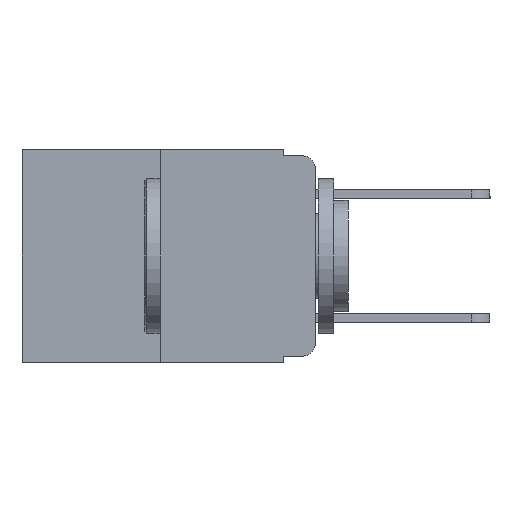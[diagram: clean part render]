
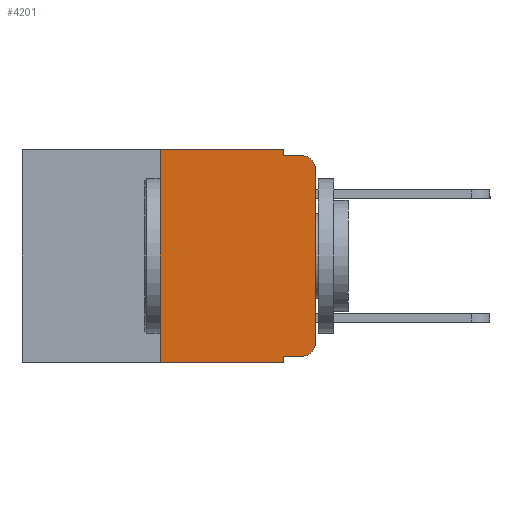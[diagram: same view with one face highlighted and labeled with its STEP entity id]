
A CAD part, left-side view. The second image highlights one B-rep face of the part: STEP entity #4201.
In plain terms, the highlighted planar face has unit normal (-1, 0, 0).
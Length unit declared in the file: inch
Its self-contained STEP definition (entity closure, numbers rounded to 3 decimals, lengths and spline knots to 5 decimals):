
#99 = DIRECTION ( 'NONE',  ( 0., -1., 0. ) ) ;
#253 = DIRECTION ( 'NONE',  ( -1., 0., 0. ) ) ;
#436 = CARTESIAN_POINT ( 'NONE',  ( 0., 0.02, -0.03 ) ) ;
#542 = ORIENTED_EDGE ( 'NONE', *, *, #10920, .F. ) ;
#738 = CARTESIAN_POINT ( 'NONE',  ( 0., 0.051, 0. ) ) ;
#1209 = CARTESIAN_POINT ( 'NONE',  ( 0., 0.473, -0.343 ) ) ;
#1216 = CARTESIAN_POINT ( 'NONE',  ( 0., 0.02, -0.01 ) ) ;
#1222 = DIRECTION ( 'NONE',  ( 0., 0., -1. ) ) ;
#1308 = ORIENTED_EDGE ( 'NONE', *, *, #7021, .T. ) ;
#1904 = LINE ( 'NONE', #7914, #5536 ) ;
#2369 = CARTESIAN_POINT ( 'NONE',  ( 0., 0.051, 0. ) ) ;
#2874 = CARTESIAN_POINT ( 'NONE',  ( 0., 0.02, -0.313 ) ) ;
#2912 = AXIS2_PLACEMENT_3D ( 'NONE', #436, #253, #1222 ) ;
#3147 = ORIENTED_EDGE ( 'NONE', *, *, #16423, .F. ) ;
#3203 = ORIENTED_EDGE ( 'NONE', *, *, #19308, .F. ) ;
#3329 = VECTOR ( 'NONE', #14555, 39.37008 ) ;
#3749 = EDGE_CURVE ( 'NONE', #11723, #16926, #11195, .T. ) ;
#3936 = DIRECTION ( 'NONE',  ( 0., -1., 0. ) ) ;
#4201 = ADVANCED_FACE ( 'NONE', ( #15948 ), #7211, .F. ) ;
#4256 = ORIENTED_EDGE ( 'NONE', *, *, #14523, .T. ) ;
#4447 = DIRECTION ( 'NONE',  ( 0., 0., -1. ) ) ;
#4767 = AXIS2_PLACEMENT_3D ( 'NONE', #2874, #13539, #4447 ) ;
#5006 = CIRCLE ( 'NONE', #2912, 0.02 ) ;
#5343 = ORIENTED_EDGE ( 'NONE', *, *, #10565, .F. ) ;
#5536 = VECTOR ( 'NONE', #99, 39.37008 ) ;
#5623 = ORIENTED_EDGE ( 'NONE', *, *, #9549, .T. ) ;
#5630 = ORIENTED_EDGE ( 'NONE', *, *, #7796, .T. ) ;
#5856 = VERTEX_POINT ( 'NONE', #1216 ) ;
#6713 = AXIS2_PLACEMENT_3D ( 'NONE', #8072, #7779, #13827 ) ;
#6740 = DIRECTION ( 'NONE',  ( 0., -1., 0. ) ) ;
#7021 = EDGE_CURVE ( 'NONE', #16243, #13256, #19217, .T. ) ;
#7211 = PLANE ( 'NONE',  #6713 ) ;
#7239 = VERTEX_POINT ( 'NONE', #8903 ) ;
#7547 = VERTEX_POINT ( 'NONE', #18936 ) ;
#7779 = DIRECTION ( 'NONE',  ( 1., 0., 0. ) ) ;
#7796 = EDGE_CURVE ( 'NONE', #13256, #5856, #5006, .T. ) ;
#7892 = VECTOR ( 'NONE', #10334, 39.37008 ) ;
#7914 = CARTESIAN_POINT ( 'NONE',  ( 0., 0.473, 0. ) ) ;
#8072 = CARTESIAN_POINT ( 'NONE',  ( 0., 0.473, 0. ) ) ;
#8608 = ORIENTED_EDGE ( 'NONE', *, *, #3749, .T. ) ;
#8821 = ORIENTED_EDGE ( 'NONE', *, *, #18351, .F. ) ;
#8903 = CARTESIAN_POINT ( 'NONE',  ( 0., 0.051, -0.01 ) ) ;
#9040 = VECTOR ( 'NONE', #12031, 39.37008 ) ;
#9549 = EDGE_CURVE ( 'NONE', #10768, #16243, #13540, .T. ) ;
#10184 = CARTESIAN_POINT ( 'NONE',  ( 0., 0., 0. ) ) ;
#10334 = DIRECTION ( 'NONE',  ( 0., 0., 1. ) ) ;
#10517 = CARTESIAN_POINT ( 'NONE',  ( 0., 0.051, 0. ) ) ;
#10565 = EDGE_CURVE ( 'NONE', #7239, #5856, #13203, .T. ) ;
#10572 = CARTESIAN_POINT ( 'NONE',  ( 0., 0.051, -0.333 ) ) ;
#10764 = CARTESIAN_POINT ( 'NONE',  ( 0., 0.25, 0. ) ) ;
#10768 = VERTEX_POINT ( 'NONE', #19278 ) ;
#10920 = EDGE_CURVE ( 'NONE', #7547, #18651, #1904, .T. ) ;
#11195 = LINE ( 'NONE', #1209, #18882 ) ;
#11723 = VERTEX_POINT ( 'NONE', #18723 ) ;
#12031 = DIRECTION ( 'NONE',  ( 0., 0., -1. ) ) ;
#12369 = VECTOR ( 'NONE', #18003, 39.37008 ) ;
#12742 = VECTOR ( 'NONE', #3936, 39.37008 ) ;
#13203 = LINE ( 'NONE', #15898, #12742 ) ;
#13256 = VERTEX_POINT ( 'NONE', #14389 ) ;
#13274 = LINE ( 'NONE', #10764, #12369 ) ;
#13539 = DIRECTION ( 'NONE',  ( -1., 0., 0. ) ) ;
#13540 = CIRCLE ( 'NONE', #4767, 0.02 ) ;
#13827 = DIRECTION ( 'NONE',  ( 0., 0., -1. ) ) ;
#14389 = CARTESIAN_POINT ( 'NONE',  ( 0., 0., -0.03 ) ) ;
#14523 = EDGE_CURVE ( 'NONE', #17809, #10768, #14627, .T. ) ;
#14555 = DIRECTION ( 'NONE',  ( 0., 0., -1. ) ) ;
#14627 = LINE ( 'NONE', #16835, #18418 ) ;
#15648 = CARTESIAN_POINT ( 'NONE',  ( 0., 0.051, -0.343 ) ) ;
#15898 = CARTESIAN_POINT ( 'NONE',  ( 0., 0.051, -0.01 ) ) ;
#15948 = FACE_OUTER_BOUND ( 'NONE', #17210, .T. ) ;
#16243 = VERTEX_POINT ( 'NONE', #18313 ) ;
#16292 = LINE ( 'NONE', #2369, #3329 ) ;
#16402 = LINE ( 'NONE', #10517, #9040 ) ;
#16423 = EDGE_CURVE ( 'NONE', #17809, #16926, #16292, .T. ) ;
#16774 = DIRECTION ( 'NONE',  ( 0., -1., 0. ) ) ;
#16835 = CARTESIAN_POINT ( 'NONE',  ( 0., 0.051, -0.333 ) ) ;
#16926 = VERTEX_POINT ( 'NONE', #15648 ) ;
#17210 = EDGE_LOOP ( 'NONE', ( #1308, #5630, #5343, #3203, #542, #8821, #8608, #3147, #4256, #5623 ) ) ;
#17809 = VERTEX_POINT ( 'NONE', #10572 ) ;
#18003 = DIRECTION ( 'NONE',  ( 0., 0., 1. ) ) ;
#18313 = CARTESIAN_POINT ( 'NONE',  ( 0., 0., -0.313 ) ) ;
#18351 = EDGE_CURVE ( 'NONE', #11723, #7547, #13274, .T. ) ;
#18418 = VECTOR ( 'NONE', #16774, 39.37008 ) ;
#18651 = VERTEX_POINT ( 'NONE', #738 ) ;
#18723 = CARTESIAN_POINT ( 'NONE',  ( 0., 0.25, -0.343 ) ) ;
#18882 = VECTOR ( 'NONE', #6740, 39.37008 ) ;
#18936 = CARTESIAN_POINT ( 'NONE',  ( 0., 0.25, 0. ) ) ;
#19217 = LINE ( 'NONE', #10184, #7892 ) ;
#19278 = CARTESIAN_POINT ( 'NONE',  ( 0., 0.02, -0.333 ) ) ;
#19308 = EDGE_CURVE ( 'NONE', #18651, #7239, #16402, .T. ) ;
